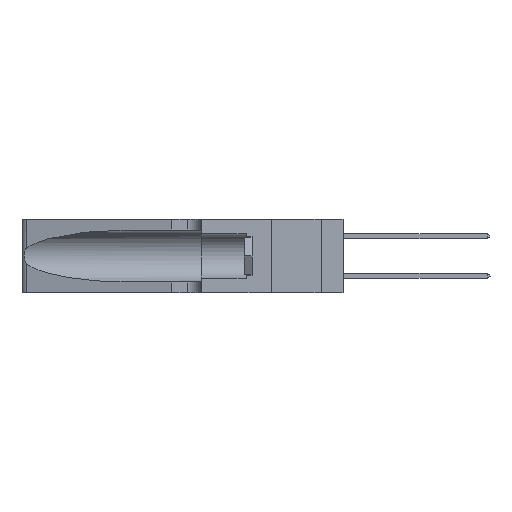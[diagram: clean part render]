
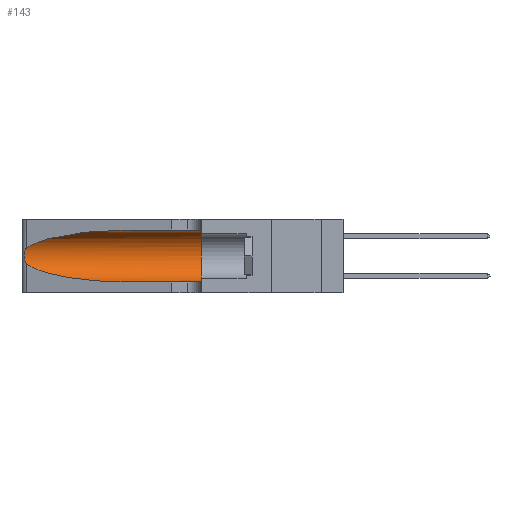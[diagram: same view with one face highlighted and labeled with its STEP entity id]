
A CAD part, left-side view. The second image highlights one B-rep face of the part: STEP entity #143.
In plain terms, the highlighted cylindrical face has radius 3.308 mm (diameter 6.617 mm), a partial arc.
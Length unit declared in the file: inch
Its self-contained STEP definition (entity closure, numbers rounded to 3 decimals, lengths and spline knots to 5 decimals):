
#143 = ADVANCED_FACE ( 'NONE', ( #4785 ), #11498, .F. ) ;
#526 = VERTEX_POINT ( 'NONE', #16214 ) ;
#620 = CARTESIAN_POINT ( 'NONE',  ( 0.1305, 1.61858, 0.31525 ) ) ;
#821 = CARTESIAN_POINT ( 'NONE',  ( 0.26075, 1.23896, 0.19203 ) ) ;
#989 = CARTESIAN_POINT ( 'NONE',  ( 0.25639, 1.23186, 0.15144 ) ) ;
#2760 = EDGE_LOOP ( 'NONE', ( #4420, #3337, #2801, #32943, #22682, #24248 ) ) ;
#2801 = ORIENTED_EDGE ( 'NONE', *, *, #33502, .T. ) ;
#2923 = CARTESIAN_POINT ( 'NONE',  ( 0.1305, 1.61858, 0.185 ) ) ;
#3337 = ORIENTED_EDGE ( 'NONE', *, *, #33958, .T. ) ;
#4107 = CARTESIAN_POINT ( 'NONE',  ( 0.25487, 1.22718, 0.14631 ) ) ;
#4327 = B_SPLINE_CURVE_WITH_KNOTS ( 'NONE', 3,
 ( #25770, #8164, #8323, #32946, #18649, #26227, #821, #4595, #40420, #4745, #11311, #989, #14885, #4107 ),
 .UNSPECIFIED., .F., .F.,
 ( 4, 2, 2, 2, 2, 2, 4 ),
 ( 0., 0.00027, 0.00053, 0.00107, 0.0016, 0.00187, 0.00214 ),
 .UNSPECIFIED. ) ;
#4420 = ORIENTED_EDGE ( 'NONE', *, *, #17006, .T. ) ;
#4595 = CARTESIAN_POINT ( 'NONE',  ( 0.26075, 1.23896, 0.178 ) ) ;
#4625 = CARTESIAN_POINT ( 'NONE',  ( 0.25487, 1.22718, 0.22369 ) ) ;
#4745 = CARTESIAN_POINT ( 'NONE',  ( 0.25856, 1.23593, 0.16098 ) ) ;
#4785 = FACE_OUTER_BOUND ( 'NONE', #2760, .T. ) ;
#4993 = VECTOR ( 'NONE', #11886, 39.37008 ) ;
#5240 = CARTESIAN_POINT ( 'NONE',  ( 0.25487, 1.22718, 0.14631 ) ) ;
#5912 = VERTEX_POINT ( 'NONE', #31901 ) ;
#8164 = CARTESIAN_POINT ( 'NONE',  ( 0.25555, 1.22994, 0.2215 ) ) ;
#8323 = CARTESIAN_POINT ( 'NONE',  ( 0.25639, 1.23184, 0.21858 ) ) ;
#11311 = CARTESIAN_POINT ( 'NONE',  ( 0.25789, 1.23486, 0.15765 ) ) ;
#11498 = CYLINDRICAL_SURFACE ( 'NONE', #31235, 0.13025 ) ;
#11886 = DIRECTION ( 'NONE',  ( 0., -1., 0. ) ) ;
#12457 = CARTESIAN_POINT ( 'NONE',  ( 0.2373, 1.15595, 0.08982 ) ) ;
#14183 = EDGE_CURVE ( 'NONE', #25112, #5912, #43268, .T. ) ;
#14378 = CARTESIAN_POINT ( 'NONE',  ( 0.1305, 0.35, 0.31525 ) ) ;
#14885 = CARTESIAN_POINT ( 'NONE',  ( 0.25555, 1.22993, 0.14849 ) ) ;
#16214 = CARTESIAN_POINT ( 'NONE',  ( 0.1305, 0.72297, 0.31525 ) ) ;
#17006 = EDGE_CURVE ( 'NONE', #526, #40392, #24442, .T. ) ;
#17175 = VECTOR ( 'NONE', #46106, 39.37008 ) ;
#17633 = CARTESIAN_POINT ( 'NONE',  ( 0.1305, 1.61858, 0.05475 ) ) ;
#18399 = CARTESIAN_POINT ( 'NONE',  ( 0.25487, 1.22718, 0.14631 ) ) ;
#18649 = CARTESIAN_POINT ( 'NONE',  ( 0.25854, 1.2359, 0.20912 ) ) ;
#19158 = CARTESIAN_POINT ( 'NONE',  ( 0.18966, 0.96281, 0.31525 ) ) ;
#20939 =( BOUNDED_CURVE ( )  B_SPLINE_CURVE ( 3, ( #5240, #12457, #45132, #34255 ),
 .UNSPECIFIED., .F., .T. ) 
 B_SPLINE_CURVE_WITH_KNOTS ( ( 4, 4 ),
 ( 3.44316, 4.71239 ),
 .UNSPECIFIED. ) 
 CURVE ( )  GEOMETRIC_REPRESENTATION_ITEM ( )  RATIONAL_B_SPLINE_CURVE ( ( 1., 0.87, 0.87, 1. ) ) 
 REPRESENTATION_ITEM ( '' )  );
#20994 = VERTEX_POINT ( 'NONE', #18399 ) ;
#22179 = AXIS2_PLACEMENT_3D ( 'NONE', #27732, #45840, #34649 ) ;
#22682 = ORIENTED_EDGE ( 'NONE', *, *, #14183, .F. ) ;
#23945 = LINE ( 'NONE', #17633, #17175 ) ;
#24110 = DIRECTION ( 'NONE',  ( 0., -1., 0. ) ) ;
#24248 = ORIENTED_EDGE ( 'NONE', *, *, #25152, .F. ) ;
#24442 =( BOUNDED_CURVE ( )  B_SPLINE_CURVE ( 3, ( #29523, #19158, #36878, #4625 ),
 .UNSPECIFIED., .F., .T. ) 
 B_SPLINE_CURVE_WITH_KNOTS ( ( 4, 4 ),
 ( 1.5708, 2.84003 ),
 .UNSPECIFIED. ) 
 CURVE ( )  GEOMETRIC_REPRESENTATION_ITEM ( )  RATIONAL_B_SPLINE_CURVE ( ( 1., 0.87, 0.87, 1. ) ) 
 REPRESENTATION_ITEM ( '' )  );
#25112 = VERTEX_POINT ( 'NONE', #14378 ) ;
#25152 = EDGE_CURVE ( 'NONE', #526, #25112, #32467, .T. ) ;
#25770 = CARTESIAN_POINT ( 'NONE',  ( 0.25487, 1.22718, 0.22369 ) ) ;
#26227 = CARTESIAN_POINT ( 'NONE',  ( 0.26018, 1.23835, 0.19895 ) ) ;
#27700 = DIRECTION ( 'NONE',  ( 0., 0., -1. ) ) ;
#27732 = CARTESIAN_POINT ( 'NONE',  ( 0.1305, 0.35, 0.185 ) ) ;
#28765 = VERTEX_POINT ( 'NONE', #29838 ) ;
#29523 = CARTESIAN_POINT ( 'NONE',  ( 0.1305, 0.72297, 0.31525 ) ) ;
#29838 = CARTESIAN_POINT ( 'NONE',  ( 0.1305, 0.72297, 0.05475 ) ) ;
#30992 = EDGE_CURVE ( 'NONE', #28765, #5912, #23945, .T. ) ;
#31235 = AXIS2_PLACEMENT_3D ( 'NONE', #2923, #24110, #27700 ) ;
#31901 = CARTESIAN_POINT ( 'NONE',  ( 0.1305, 0.35, 0.05475 ) ) ;
#32467 = LINE ( 'NONE', #620, #4993 ) ;
#32943 = ORIENTED_EDGE ( 'NONE', *, *, #30992, .T. ) ;
#32946 = CARTESIAN_POINT ( 'NONE',  ( 0.25787, 1.23484, 0.2124 ) ) ;
#33502 = EDGE_CURVE ( 'NONE', #20994, #28765, #20939, .T. ) ;
#33958 = EDGE_CURVE ( 'NONE', #40392, #20994, #4327, .T. ) ;
#34255 = CARTESIAN_POINT ( 'NONE',  ( 0.1305, 0.72297, 0.05475 ) ) ;
#34649 = DIRECTION ( 'NONE',  ( 0., 0., 1. ) ) ;
#36878 = CARTESIAN_POINT ( 'NONE',  ( 0.2373, 1.15595, 0.28018 ) ) ;
#40392 = VERTEX_POINT ( 'NONE', #41346 ) ;
#40420 = CARTESIAN_POINT ( 'NONE',  ( 0.26017, 1.23833, 0.17102 ) ) ;
#41346 = CARTESIAN_POINT ( 'NONE',  ( 0.25487, 1.22718, 0.22369 ) ) ;
#43268 = CIRCLE ( 'NONE', #22179, 0.13025 ) ;
#45132 = CARTESIAN_POINT ( 'NONE',  ( 0.18966, 0.96281, 0.05475 ) ) ;
#45840 = DIRECTION ( 'NONE',  ( 0., 1., 0. ) ) ;
#46106 = DIRECTION ( 'NONE',  ( 0., -1., 0. ) ) ;
